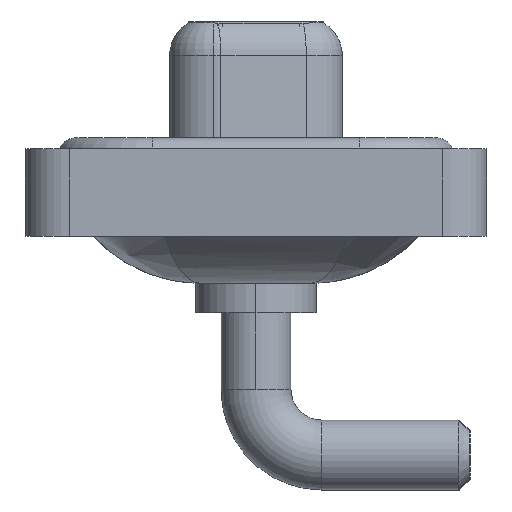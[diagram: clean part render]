
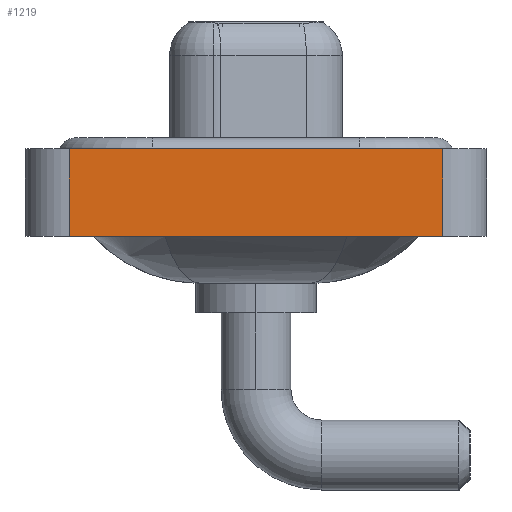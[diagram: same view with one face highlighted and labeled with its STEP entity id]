
A CAD part, left-side view. The second image highlights one B-rep face of the part: STEP entity #1219.
In plain terms, the highlighted planar face has unit normal (-1, 0, 0).
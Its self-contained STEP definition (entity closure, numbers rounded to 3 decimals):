
#237 = LINE ( 'NONE', #10947, #15199 ) ;
#243 = CARTESIAN_POINT ( 'NONE',  ( -7.3, -8.55, -3.6 ) ) ;
#1150 = EDGE_CURVE ( 'NONE', #7521, #17124, #237, .T. ) ;
#1219 = ADVANCED_FACE ( 'NONE', ( #1644 ), #10061, .T. ) ;
#1532 = VECTOR ( 'NONE', #10914, 1000. ) ;
#1644 = FACE_OUTER_BOUND ( 'NONE', #1946, .T. ) ;
#1946 = EDGE_LOOP ( 'NONE', ( #14140, #15442, #4223, #14426 ) ) ;
#2031 = CARTESIAN_POINT ( 'NONE',  ( -7.3, 8.55, -3.6 ) ) ;
#2830 = CARTESIAN_POINT ( 'NONE',  ( -7.3, -8.55, 0.4 ) ) ;
#3153 = DIRECTION ( 'NONE',  ( 0., 0., 1. ) ) ;
#3331 = DIRECTION ( 'NONE',  ( -1., 0., 0. ) ) ;
#3941 = VECTOR ( 'NONE', #15589, 1000. ) ;
#4223 = ORIENTED_EDGE ( 'NONE', *, *, #6748, .F. ) ;
#4484 = CARTESIAN_POINT ( 'NONE',  ( -7.3, -8.55, -3.6 ) ) ;
#4790 = CARTESIAN_POINT ( 'NONE',  ( -7.3, -8.55, 0.4 ) ) ;
#5251 = LINE ( 'NONE', #10742, #1532 ) ;
#5385 = VERTEX_POINT ( 'NONE', #14774 ) ;
#6544 = EDGE_CURVE ( 'NONE', #17124, #13410, #10490, .T. ) ;
#6707 = AXIS2_PLACEMENT_3D ( 'NONE', #4484, #3331, #3153 ) ;
#6748 = EDGE_CURVE ( 'NONE', #7521, #5385, #5251, .T. ) ;
#7521 = VERTEX_POINT ( 'NONE', #2031 ) ;
#9623 = DIRECTION ( 'NONE',  ( 0., -1., 0. ) ) ;
#10061 = PLANE ( 'NONE',  #6707 ) ;
#10196 = LINE ( 'NONE', #4790, #11803 ) ;
#10490 = LINE ( 'NONE', #12951, #3941 ) ;
#10742 = CARTESIAN_POINT ( 'NONE',  ( -7.3, 8.55, -3.6 ) ) ;
#10914 = DIRECTION ( 'NONE',  ( 0., 0., 1. ) ) ;
#10947 = CARTESIAN_POINT ( 'NONE',  ( -7.3, -8.55, -3.6 ) ) ;
#11803 = VECTOR ( 'NONE', #12918, 1000. ) ;
#12918 = DIRECTION ( 'NONE',  ( 0., -1., 0. ) ) ;
#12951 = CARTESIAN_POINT ( 'NONE',  ( -7.3, -8.55, -3.6 ) ) ;
#13410 = VERTEX_POINT ( 'NONE', #2830 ) ;
#14140 = ORIENTED_EDGE ( 'NONE', *, *, #6544, .T. ) ;
#14426 = ORIENTED_EDGE ( 'NONE', *, *, #1150, .T. ) ;
#14774 = CARTESIAN_POINT ( 'NONE',  ( -7.3, 8.55, 0.4 ) ) ;
#15199 = VECTOR ( 'NONE', #9623, 1000. ) ;
#15442 = ORIENTED_EDGE ( 'NONE', *, *, #16347, .F. ) ;
#15589 = DIRECTION ( 'NONE',  ( 0., 0., 1. ) ) ;
#16347 = EDGE_CURVE ( 'NONE', #5385, #13410, #10196, .T. ) ;
#17124 = VERTEX_POINT ( 'NONE', #243 ) ;
